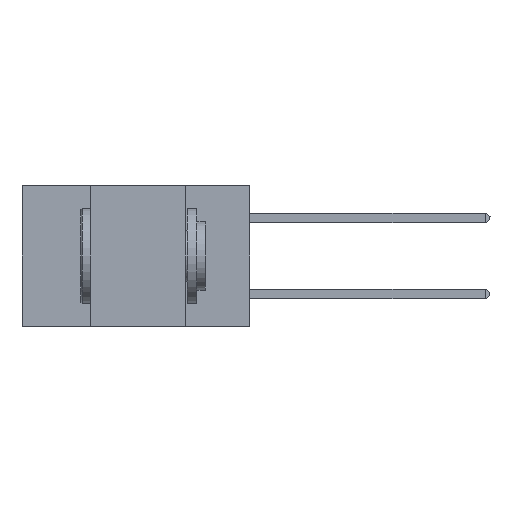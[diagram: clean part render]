
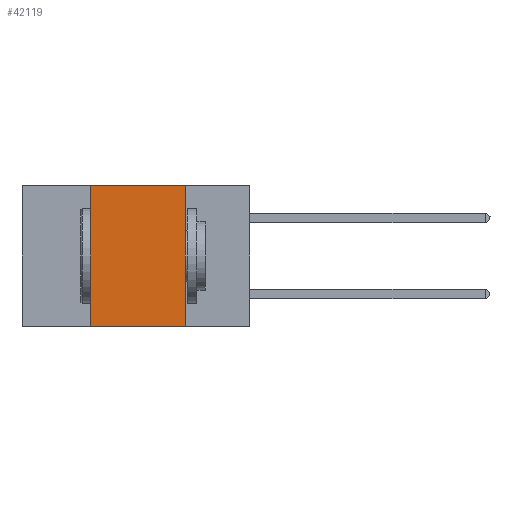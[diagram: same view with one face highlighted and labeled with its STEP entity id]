
A CAD part, left-side view. The second image highlights one B-rep face of the part: STEP entity #42119.
In plain terms, the highlighted planar face has unit normal (-1, 0, 0).
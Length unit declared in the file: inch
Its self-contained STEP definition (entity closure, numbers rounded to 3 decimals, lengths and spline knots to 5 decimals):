
#1349 = LINE ( 'NONE', #45672, #19421 ) ;
#3917 = EDGE_LOOP ( 'NONE', ( #43323, #45676, #32117, #34290 ) ) ;
#4168 = EDGE_CURVE ( 'NONE', #11168, #32957, #33521, .T. ) ;
#5727 = AXIS2_PLACEMENT_3D ( 'NONE', #30890, #38181, #16507 ) ;
#5823 = VECTOR ( 'NONE', #36531, 39.37008 ) ;
#6425 = VERTEX_POINT ( 'NONE', #37722 ) ;
#7249 = VERTEX_POINT ( 'NONE', #31623 ) ;
#7886 = EDGE_CURVE ( 'NONE', #11168, #7249, #1349, .T. ) ;
#10610 = VECTOR ( 'NONE', #43174, 39.37008 ) ;
#11168 = VERTEX_POINT ( 'NONE', #36070 ) ;
#13791 = DIRECTION ( 'NONE',  ( 0., -1., 0. ) ) ;
#15365 = FACE_OUTER_BOUND ( 'NONE', #3917, .T. ) ;
#16507 = DIRECTION ( 'NONE',  ( 0., 0., -1. ) ) ;
#16901 = LINE ( 'NONE', #31789, #31588 ) ;
#19421 = VECTOR ( 'NONE', #42029, 39.37008 ) ;
#21975 = CARTESIAN_POINT ( 'NONE',  ( 0., 0.6, -0.37 ) ) ;
#30116 = CARTESIAN_POINT ( 'NONE',  ( 0., 0.17, -0.37 ) ) ;
#30890 = CARTESIAN_POINT ( 'NONE',  ( 0., 0.6, 0. ) ) ;
#31588 = VECTOR ( 'NONE', #13791, 39.37008 ) ;
#31623 = CARTESIAN_POINT ( 'NONE',  ( 0., 0.42, 0. ) ) ;
#31789 = CARTESIAN_POINT ( 'NONE',  ( 0., 0.6, 0. ) ) ;
#32117 = ORIENTED_EDGE ( 'NONE', *, *, #7886, .F. ) ;
#32957 = VERTEX_POINT ( 'NONE', #30116 ) ;
#33521 = LINE ( 'NONE', #21975, #5823 ) ;
#34290 = ORIENTED_EDGE ( 'NONE', *, *, #4168, .T. ) ;
#36070 = CARTESIAN_POINT ( 'NONE',  ( 0., 0.42, -0.37 ) ) ;
#36531 = DIRECTION ( 'NONE',  ( 0., -1., 0. ) ) ;
#37722 = CARTESIAN_POINT ( 'NONE',  ( 0., 0.17, 0. ) ) ;
#38181 = DIRECTION ( 'NONE',  ( 1., 0., 0. ) ) ;
#38964 = EDGE_CURVE ( 'NONE', #7249, #6425, #16901, .T. ) ;
#39449 = LINE ( 'NONE', #39560, #10610 ) ;
#39560 = CARTESIAN_POINT ( 'NONE',  ( 0., 0.17, 0. ) ) ;
#42029 = DIRECTION ( 'NONE',  ( 0., 0., 1. ) ) ;
#42119 = ADVANCED_FACE ( 'NONE', ( #15365 ), #45297, .F. ) ;
#43174 = DIRECTION ( 'NONE',  ( 0., 0., -1. ) ) ;
#43323 = ORIENTED_EDGE ( 'NONE', *, *, #44434, .F. ) ;
#44434 = EDGE_CURVE ( 'NONE', #6425, #32957, #39449, .T. ) ;
#45297 = PLANE ( 'NONE',  #5727 ) ;
#45672 = CARTESIAN_POINT ( 'NONE',  ( 0., 0.42, 0. ) ) ;
#45676 = ORIENTED_EDGE ( 'NONE', *, *, #38964, .F. ) ;
